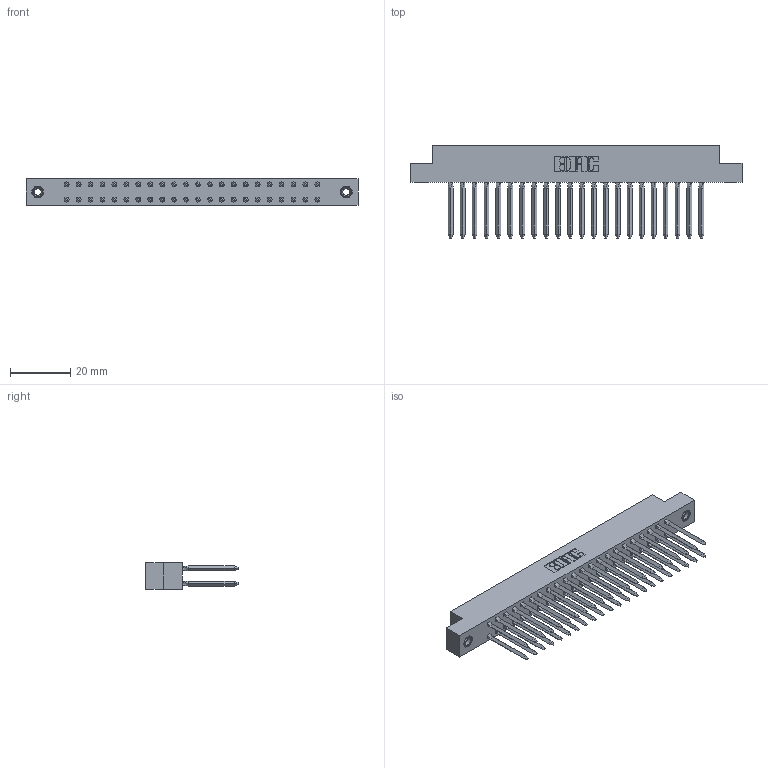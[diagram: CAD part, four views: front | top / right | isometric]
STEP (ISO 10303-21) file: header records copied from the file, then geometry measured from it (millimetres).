
FILE_DESCRIPTION (( 'STEP AP203' ), '1' );
FILE_NAME ('338-044-541-208.STEP', '2020-03-24T18:42:24', ( '' ), ( '' ), 'SwSTEP 2.0', 'SolidWorks 2016', '' );
FILE_SCHEMA (( 'CONFIG_CONTROL_DESIGN' ));
Length unit declared in the file: inch
Products named in the file (4): 338-044-541-208; 338-210-001_338-210-022-004; 338-290-001_541; 345-250-001_345-250-003-102
Assembly tree (47 placements, depth 2):
  338-044-541-208
    338-210-001_338-210-022-004
    338-290-001_541  x44
    345-250-001_345-250-003-102  x2
Bounding box: 110.19 x 30.56 x 8.71 mm (x, y, z)
Volume: 8456.7 mm3; surface area: 15664.3 mm2
Topology: 47 solids, 47 shells, 3102 faces, 8307 edges, 5266 vertices
Faces by surface type: plane 2150, cylinder 760, bspline 176, cone 12, torus 4
Entity records: 46165 total; most frequent: CARTESIAN_POINT 9123, ORIENTED_EDGE 7656, DIRECTION 7201, EDGE_CURVE 3828, VECTOR 2845, LINE 2845, VERTEX_POINT 2484, AXIS2_PLACEMENT_3D 2178
